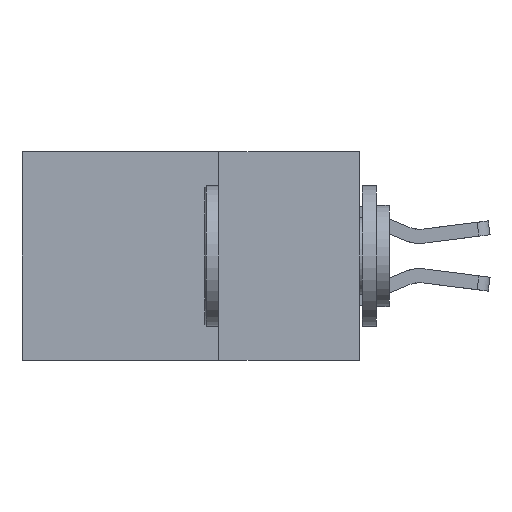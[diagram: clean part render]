
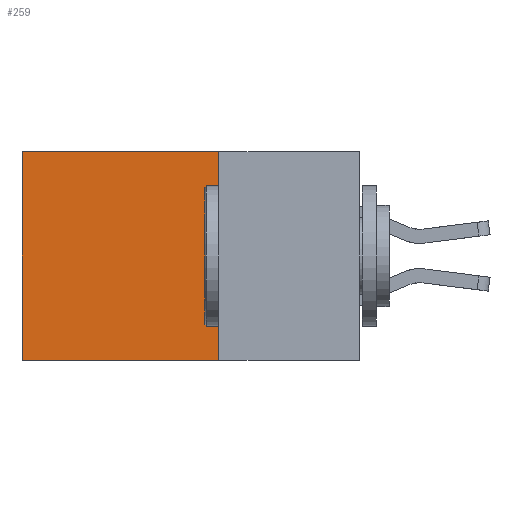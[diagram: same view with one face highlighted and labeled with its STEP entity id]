
A CAD part, left-side view. The second image highlights one B-rep face of the part: STEP entity #259.
In plain terms, the highlighted planar face has unit normal (-1, 0, 0).
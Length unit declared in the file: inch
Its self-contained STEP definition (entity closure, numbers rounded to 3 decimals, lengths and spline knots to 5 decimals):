
#259 = ADVANCED_FACE ( 'NONE', ( #6851 ), #1233, .F. ) ;
#414 = EDGE_CURVE ( 'NONE', #1705, #5594, #9986, .T. ) ;
#776 = VECTOR ( 'NONE', #4471, 39.37008 ) ;
#1233 = PLANE ( 'NONE',  #9541 ) ;
#1301 = CARTESIAN_POINT ( 'NONE',  ( 0.2875, 0.25, -0.37 ) ) ;
#1460 = CARTESIAN_POINT ( 'NONE',  ( 0.2875, 0.25, 0. ) ) ;
#1705 = VERTEX_POINT ( 'NONE', #9247 ) ;
#1886 = DIRECTION ( 'NONE',  ( 0., 1., 0. ) ) ;
#2115 = LINE ( 'NONE', #4380, #776 ) ;
#2265 = LINE ( 'NONE', #2514, #12281 ) ;
#2405 = EDGE_CURVE ( 'NONE', #10096, #1705, #2265, .T. ) ;
#2432 = CARTESIAN_POINT ( 'NONE',  ( 0.2875, 0.25, -0.37 ) ) ;
#2514 = CARTESIAN_POINT ( 'NONE',  ( 0.2875, 0.25, 0. ) ) ;
#2784 = DIRECTION ( 'NONE',  ( 0., 0., -1. ) ) ;
#2919 = VECTOR ( 'NONE', #11957, 39.37008 ) ;
#3065 = DIRECTION ( 'NONE',  ( 0., 0., -1. ) ) ;
#3177 = EDGE_CURVE ( 'NONE', #10096, #8232, #2115, .T. ) ;
#3334 = ORIENTED_EDGE ( 'NONE', *, *, #10581, .F. ) ;
#4380 = CARTESIAN_POINT ( 'NONE',  ( 0.2875, 0.25, 0. ) ) ;
#4471 = DIRECTION ( 'NONE',  ( 0., 0., -1. ) ) ;
#5594 = VERTEX_POINT ( 'NONE', #11845 ) ;
#5875 = ORIENTED_EDGE ( 'NONE', *, *, #414, .T. ) ;
#6018 = CARTESIAN_POINT ( 'NONE',  ( 0.2875, 0.25, 0. ) ) ;
#6277 = LINE ( 'NONE', #2432, #2919 ) ;
#6851 = FACE_OUTER_BOUND ( 'NONE', #9555, .T. ) ;
#8003 = DIRECTION ( 'NONE',  ( 1., 0., 0. ) ) ;
#8061 = VECTOR ( 'NONE', #2784, 39.37008 ) ;
#8232 = VERTEX_POINT ( 'NONE', #1301 ) ;
#9247 = CARTESIAN_POINT ( 'NONE',  ( 0.2875, 0.6, 0. ) ) ;
#9541 = AXIS2_PLACEMENT_3D ( 'NONE', #6018, #8003, #3065 ) ;
#9544 = ORIENTED_EDGE ( 'NONE', *, *, #3177, .F. ) ;
#9555 = EDGE_LOOP ( 'NONE', ( #5875, #3334, #9544, #11635 ) ) ;
#9746 = CARTESIAN_POINT ( 'NONE',  ( 0.2875, 0.6, 0. ) ) ;
#9986 = LINE ( 'NONE', #9746, #8061 ) ;
#10096 = VERTEX_POINT ( 'NONE', #1460 ) ;
#10581 = EDGE_CURVE ( 'NONE', #8232, #5594, #6277, .T. ) ;
#11635 = ORIENTED_EDGE ( 'NONE', *, *, #2405, .T. ) ;
#11845 = CARTESIAN_POINT ( 'NONE',  ( 0.2875, 0.6, -0.37 ) ) ;
#11957 = DIRECTION ( 'NONE',  ( 0., 1., 0. ) ) ;
#12281 = VECTOR ( 'NONE', #1886, 39.37008 ) ;
